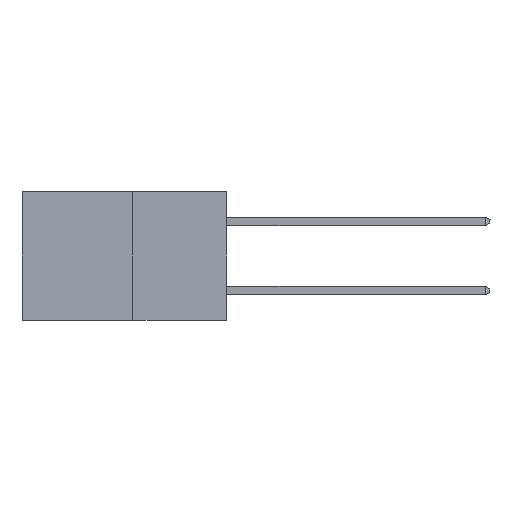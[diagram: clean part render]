
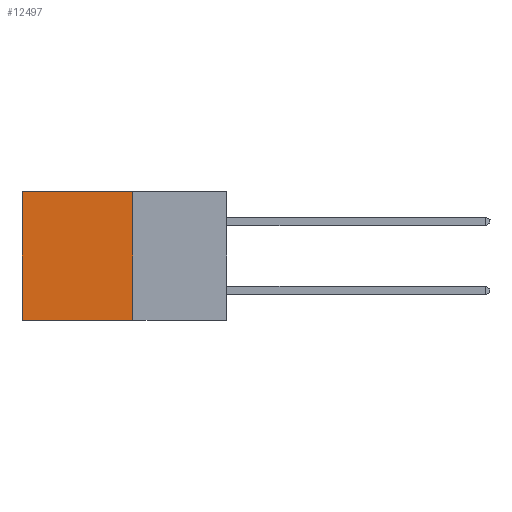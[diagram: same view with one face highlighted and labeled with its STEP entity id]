
A CAD part, left-side view. The second image highlights one B-rep face of the part: STEP entity #12497.
In plain terms, the highlighted planar face has unit normal (-1, 0, 0).
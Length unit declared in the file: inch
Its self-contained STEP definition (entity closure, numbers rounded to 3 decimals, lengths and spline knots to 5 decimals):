
#21 = DIRECTION ( 'NONE',  ( 0., 1., 0. ) ) ;
#1132 = EDGE_CURVE ( 'NONE', #19291, #8782, #18842, .T. ) ;
#2064 = ORIENTED_EDGE ( 'NONE', *, *, #14220, .T. ) ;
#2189 = LINE ( 'NONE', #6466, #5964 ) ;
#3043 = EDGE_CURVE ( 'NONE', #19291, #12574, #3959, .T. ) ;
#3390 = VERTEX_POINT ( 'NONE', #4134 ) ;
#3959 = LINE ( 'NONE', #10953, #11862 ) ;
#4134 = CARTESIAN_POINT ( 'NONE',  ( 0.277, 0.59, -0.37 ) ) ;
#5964 = VECTOR ( 'NONE', #7031, 39.37008 ) ;
#6009 = VECTOR ( 'NONE', #18035, 39.37008 ) ;
#6466 = CARTESIAN_POINT ( 'NONE',  ( 0.277, 0.59, -0.37 ) ) ;
#7031 = DIRECTION ( 'NONE',  ( 0., 0., -1. ) ) ;
#7094 = DIRECTION ( 'NONE',  ( 1., 0., 0. ) ) ;
#7233 = CARTESIAN_POINT ( 'NONE',  ( 0.277, 0.27, -0.37 ) ) ;
#7863 = EDGE_CURVE ( 'NONE', #12574, #3390, #13363, .T. ) ;
#8782 = VERTEX_POINT ( 'NONE', #9461 ) ;
#8844 = CARTESIAN_POINT ( 'NONE',  ( 0.277, 0.27, 0. ) ) ;
#9461 = CARTESIAN_POINT ( 'NONE',  ( 0.277, 0.59, 0. ) ) ;
#9734 = ORIENTED_EDGE ( 'NONE', *, *, #7863, .F. ) ;
#10517 = DIRECTION ( 'NONE',  ( 0., 0., -1. ) ) ;
#10953 = CARTESIAN_POINT ( 'NONE',  ( 0.277, 0.27, -0.37 ) ) ;
#11213 = PLANE ( 'NONE',  #15178 ) ;
#11862 = VECTOR ( 'NONE', #10517, 39.37008 ) ;
#11911 = DIRECTION ( 'NONE',  ( 0., 0., -1. ) ) ;
#12497 = ADVANCED_FACE ( 'NONE', ( #12668 ), #11213, .F. ) ;
#12574 = VERTEX_POINT ( 'NONE', #14032 ) ;
#12668 = FACE_OUTER_BOUND ( 'NONE', #13710, .T. ) ;
#12965 = ORIENTED_EDGE ( 'NONE', *, *, #3043, .F. ) ;
#13363 = LINE ( 'NONE', #7233, #16925 ) ;
#13710 = EDGE_LOOP ( 'NONE', ( #2064, #9734, #12965, #20052 ) ) ;
#14032 = CARTESIAN_POINT ( 'NONE',  ( 0.277, 0.27, -0.37 ) ) ;
#14220 = EDGE_CURVE ( 'NONE', #8782, #3390, #2189, .T. ) ;
#15178 = AXIS2_PLACEMENT_3D ( 'NONE', #17914, #7094, #11911 ) ;
#16925 = VECTOR ( 'NONE', #21, 39.37008 ) ;
#17914 = CARTESIAN_POINT ( 'NONE',  ( 0.277, 0.27, -0.37 ) ) ;
#18035 = DIRECTION ( 'NONE',  ( 0., 1., 0. ) ) ;
#18181 = CARTESIAN_POINT ( 'NONE',  ( 0.277, 0.27, 0. ) ) ;
#18842 = LINE ( 'NONE', #8844, #6009 ) ;
#19291 = VERTEX_POINT ( 'NONE', #18181 ) ;
#20052 = ORIENTED_EDGE ( 'NONE', *, *, #1132, .T. ) ;
